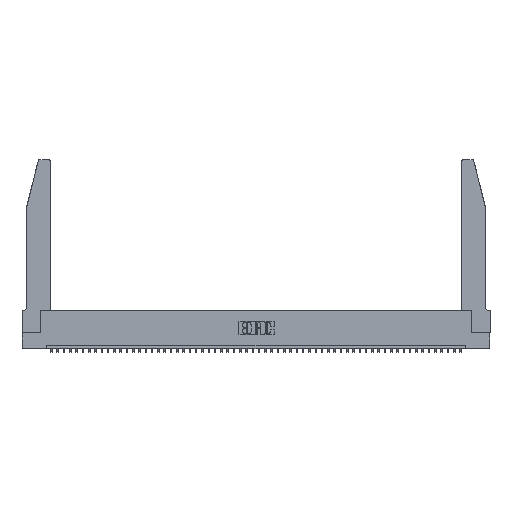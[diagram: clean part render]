
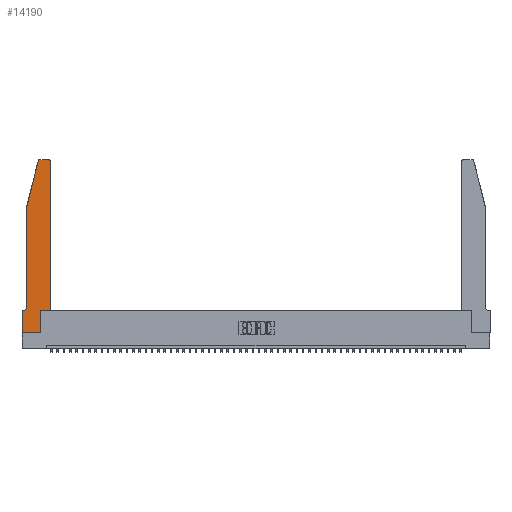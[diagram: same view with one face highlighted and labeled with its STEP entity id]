
A CAD part, top view. The second image highlights one B-rep face of the part: STEP entity #14190.
In plain terms, the highlighted planar face has unit normal (0, 0, 1).
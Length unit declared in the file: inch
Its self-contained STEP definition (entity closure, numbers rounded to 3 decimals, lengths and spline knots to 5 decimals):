
#729 = CARTESIAN_POINT ( 'NONE',  ( 0.0755, 0.42, 0.37 ) ) ;
#1199 = DIRECTION ( 'NONE',  ( 0., -1., 0. ) ) ;
#1481 = EDGE_CURVE ( 'NONE', #5898, #45763, #5165, .T. ) ;
#2044 = DIRECTION ( 'NONE',  ( -0.239, -0.971, 0. ) ) ;
#2563 = CARTESIAN_POINT ( 'NONE',  ( 0.284, 2.75, 0.37 ) ) ;
#2725 = CARTESIAN_POINT ( 'NONE',  ( 0., 0., 0.37 ) ) ;
#3055 = DIRECTION ( 'NONE',  ( 1., 0., 0. ) ) ;
#3700 = CIRCLE ( 'NONE', #7774, 0.03 ) ;
#4531 = AXIS2_PLACEMENT_3D ( 'NONE', #11187, #47214, #4933 ) ;
#4933 = DIRECTION ( 'NONE',  ( 1., 0., 0. ) ) ;
#5165 = LINE ( 'NONE', #9432, #46150 ) ;
#5213 = VECTOR ( 'NONE', #5813, 39.37008 ) ;
#5812 = DIRECTION ( 'NONE',  ( 0., 1., 0. ) ) ;
#5813 = DIRECTION ( 'NONE',  ( -1., 0., 0. ) ) ;
#5898 = VERTEX_POINT ( 'NONE', #6633 ) ;
#5973 = CARTESIAN_POINT ( 'NONE',  ( 0.2865, 0.35, 0.37 ) ) ;
#6574 = EDGE_CURVE ( 'NONE', #46715, #10632, #21928, .T. ) ;
#6633 = CARTESIAN_POINT ( 'NONE',  ( 0.25487, 2.72718, 0.37 ) ) ;
#6749 = VECTOR ( 'NONE', #1199, 39.37008 ) ;
#6855 = DIRECTION ( 'NONE',  ( 1., 0., 0. ) ) ;
#7053 = CARTESIAN_POINT ( 'NONE',  ( 0., 0., 0.37 ) ) ;
#7233 = LINE ( 'NONE', #37267, #18984 ) ;
#7765 = CARTESIAN_POINT ( 'NONE',  ( 0.4205, 2.72, 0.37 ) ) ;
#7774 = AXIS2_PLACEMENT_3D ( 'NONE', #42704, #38848, #3055 ) ;
#8075 = LINE ( 'NONE', #25645, #40919 ) ;
#8166 = LINE ( 'NONE', #11856, #12550 ) ;
#8449 = ORIENTED_EDGE ( 'NONE', *, *, #11807, .T. ) ;
#8933 = CARTESIAN_POINT ( 'NONE',  ( 0.4505, 2.72, 0.37 ) ) ;
#8939 = VERTEX_POINT ( 'NONE', #21344 ) ;
#9432 = CARTESIAN_POINT ( 'NONE',  ( 0.0755, 2., 0.37 ) ) ;
#9503 = ORIENTED_EDGE ( 'NONE', *, *, #6574, .T. ) ;
#10370 = ORIENTED_EDGE ( 'NONE', *, *, #1481, .T. ) ;
#10632 = VERTEX_POINT ( 'NONE', #2563 ) ;
#10655 = PLANE ( 'NONE',  #4531 ) ;
#10830 = CARTESIAN_POINT ( 'NONE',  ( 0.2865, 0.35, 0.37 ) ) ;
#11187 = CARTESIAN_POINT ( 'NONE',  ( 0., 0.35, 0.37 ) ) ;
#11393 = CIRCLE ( 'NONE', #47562, 0.07 ) ;
#11807 = EDGE_CURVE ( 'NONE', #8939, #13700, #34814, .T. ) ;
#11856 = CARTESIAN_POINT ( 'NONE',  ( 0.0755, 0.35, 0.37 ) ) ;
#12409 = DIRECTION ( 'NONE',  ( 1., 0., 0. ) ) ;
#12509 = AXIS2_PLACEMENT_3D ( 'NONE', #7765, #20488, #12409 ) ;
#12550 = VECTOR ( 'NONE', #15620, 39.37008 ) ;
#13700 = VERTEX_POINT ( 'NONE', #10830 ) ;
#14190 = ADVANCED_FACE ( 'NONE', ( #22302 ), #10655, .T. ) ;
#15045 = EDGE_CURVE ( 'NONE', #23401, #43488, #17201, .T. ) ;
#15620 = DIRECTION ( 'NONE',  ( -1., 0., 0. ) ) ;
#16132 = EDGE_CURVE ( 'NONE', #43488, #8939, #17091, .T. ) ;
#16203 = ORIENTED_EDGE ( 'NONE', *, *, #30178, .T. ) ;
#17091 = LINE ( 'NONE', #2725, #33214 ) ;
#17150 = DIRECTION ( 'NONE',  ( 1., 0., 0. ) ) ;
#17201 = LINE ( 'NONE', #21051, #6749 ) ;
#17693 = CARTESIAN_POINT ( 'NONE',  ( 0.0055, 0.35, 0.37 ) ) ;
#18301 = ORIENTED_EDGE ( 'NONE', *, *, #37309, .T. ) ;
#18752 = VERTEX_POINT ( 'NONE', #17693 ) ;
#18984 = VECTOR ( 'NONE', #30040, 39.37008 ) ;
#20488 = DIRECTION ( 'NONE',  ( 0., 0., 1. ) ) ;
#20594 = VERTEX_POINT ( 'NONE', #729 ) ;
#21051 = CARTESIAN_POINT ( 'NONE',  ( 0., 0., 0.37 ) ) ;
#21317 = CARTESIAN_POINT ( 'NONE',  ( 0.2605, 2.75, 0.37 ) ) ;
#21344 = CARTESIAN_POINT ( 'NONE',  ( 0.2865, 0., 0.37 ) ) ;
#21790 = DIRECTION ( 'NONE',  ( 0., 1., 0. ) ) ;
#21928 = LINE ( 'NONE', #21317, #5213 ) ;
#22302 = FACE_OUTER_BOUND ( 'NONE', #30895, .T. ) ;
#22377 = VECTOR ( 'NONE', #5812, 39.37008 ) ;
#22398 = EDGE_CURVE ( 'NONE', #20594, #18752, #11393, .T. ) ;
#22829 = LINE ( 'NONE', #45615, #33310 ) ;
#23245 = VERTEX_POINT ( 'NONE', #33041 ) ;
#23401 = VERTEX_POINT ( 'NONE', #32163 ) ;
#24155 = DIRECTION ( 'NONE',  ( 0., 0., -1. ) ) ;
#24528 = EDGE_CURVE ( 'NONE', #10632, #5898, #3700, .T. ) ;
#25645 = CARTESIAN_POINT ( 'NONE',  ( 0.4505, 0.35, 0.37 ) ) ;
#28008 = DIRECTION ( 'NONE',  ( -1., 0., 0. ) ) ;
#30040 = DIRECTION ( 'NONE',  ( 0., -1., 0. ) ) ;
#30178 = EDGE_CURVE ( 'NONE', #37871, #46715, #40107, .T. ) ;
#30895 = EDGE_LOOP ( 'NONE', ( #9503, #47659, #10370, #42005, #36838, #47035, #35072, #38031, #8449, #44502, #18301, #16203 ) ) ;
#31876 = CARTESIAN_POINT ( 'NONE',  ( 0.4205, 2.75, 0.37 ) ) ;
#32163 = CARTESIAN_POINT ( 'NONE',  ( 0., 0.35, 0.37 ) ) ;
#33041 = CARTESIAN_POINT ( 'NONE',  ( 0.4505, 0.35, 0.37 ) ) ;
#33214 = VECTOR ( 'NONE', #6855, 39.37008 ) ;
#33310 = VECTOR ( 'NONE', #21790, 39.37008 ) ;
#34814 = LINE ( 'NONE', #5973, #22377 ) ;
#35072 = ORIENTED_EDGE ( 'NONE', *, *, #15045, .T. ) ;
#36838 = ORIENTED_EDGE ( 'NONE', *, *, #22398, .T. ) ;
#37267 = CARTESIAN_POINT ( 'NONE',  ( 0.0755, 2., 0.37 ) ) ;
#37309 = EDGE_CURVE ( 'NONE', #23245, #37871, #22829, .T. ) ;
#37871 = VERTEX_POINT ( 'NONE', #8933 ) ;
#38031 = ORIENTED_EDGE ( 'NONE', *, *, #16132, .T. ) ;
#38848 = DIRECTION ( 'NONE',  ( 0., 0., 1. ) ) ;
#40107 = CIRCLE ( 'NONE', #12509, 0.03 ) ;
#40919 = VECTOR ( 'NONE', #17150, 39.37008 ) ;
#42005 = ORIENTED_EDGE ( 'NONE', *, *, #43906, .T. ) ;
#42704 = CARTESIAN_POINT ( 'NONE',  ( 0.284, 2.72, 0.37 ) ) ;
#43488 = VERTEX_POINT ( 'NONE', #7053 ) ;
#43906 = EDGE_CURVE ( 'NONE', #45763, #20594, #7233, .T. ) ;
#44502 = ORIENTED_EDGE ( 'NONE', *, *, #44568, .T. ) ;
#44568 = EDGE_CURVE ( 'NONE', #13700, #23245, #8075, .T. ) ;
#45615 = CARTESIAN_POINT ( 'NONE',  ( 0.4505, 0.35, 0.37 ) ) ;
#45763 = VERTEX_POINT ( 'NONE', #49505 ) ;
#46150 = VECTOR ( 'NONE', #2044, 39.37008 ) ;
#46715 = VERTEX_POINT ( 'NONE', #31876 ) ;
#47035 = ORIENTED_EDGE ( 'NONE', *, *, #48465, .T. ) ;
#47214 = DIRECTION ( 'NONE',  ( 0., 0., 1. ) ) ;
#47562 = AXIS2_PLACEMENT_3D ( 'NONE', #47791, #24155, #28008 ) ;
#47659 = ORIENTED_EDGE ( 'NONE', *, *, #24528, .T. ) ;
#47791 = CARTESIAN_POINT ( 'NONE',  ( 0.0055, 0.42, 0.37 ) ) ;
#48465 = EDGE_CURVE ( 'NONE', #18752, #23401, #8166, .T. ) ;
#49505 = CARTESIAN_POINT ( 'NONE',  ( 0.0755, 2., 0.37 ) ) ;
